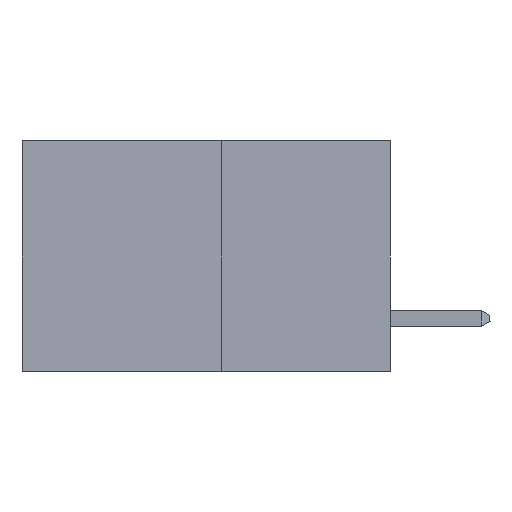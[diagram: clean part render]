
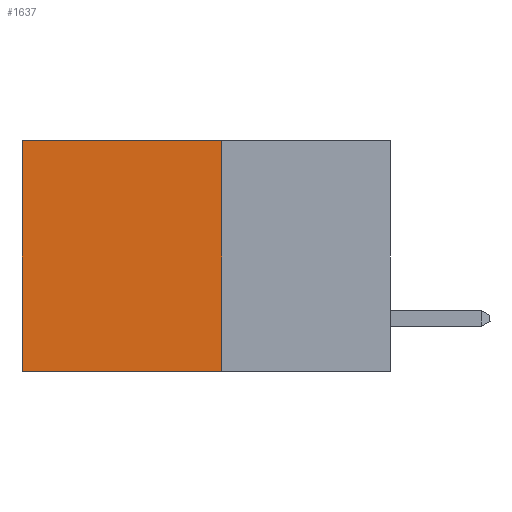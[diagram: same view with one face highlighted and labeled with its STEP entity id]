
A CAD part, left-side view. The second image highlights one B-rep face of the part: STEP entity #1637.
In plain terms, the highlighted planar face has unit normal (-1, 0, 0).
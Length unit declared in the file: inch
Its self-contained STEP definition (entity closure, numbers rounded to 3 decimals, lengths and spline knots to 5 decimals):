
#63 = EDGE_CURVE ( 'NONE', #3981, #15127, #5803, .T. ) ;
#303 = VERTEX_POINT ( 'NONE', #14389 ) ;
#711 = VECTOR ( 'NONE', #12782, 39.37008 ) ;
#761 = EDGE_LOOP ( 'NONE', ( #2103, #2134, #8928, #1982 ) ) ;
#1408 = PLANE ( 'NONE',  #7866 ) ;
#1637 = ADVANCED_FACE ( 'NONE', ( #5552 ), #1408, .F. ) ;
#1967 = VECTOR ( 'NONE', #15109, 39.37008 ) ;
#1982 = ORIENTED_EDGE ( 'NONE', *, *, #3085, .T. ) ;
#2053 = CARTESIAN_POINT ( 'NONE',  ( 0.277, 0.27, -0.37 ) ) ;
#2103 = ORIENTED_EDGE ( 'NONE', *, *, #63, .T. ) ;
#2134 = ORIENTED_EDGE ( 'NONE', *, *, #8322, .F. ) ;
#2957 = EDGE_CURVE ( 'NONE', #303, #5898, #11823, .T. ) ;
#3085 = EDGE_CURVE ( 'NONE', #303, #3981, #9901, .T. ) ;
#3717 = LINE ( 'NONE', #12818, #711 ) ;
#3981 = VERTEX_POINT ( 'NONE', #5483 ) ;
#5483 = CARTESIAN_POINT ( 'NONE',  ( 0.277, 0.59, 0. ) ) ;
#5552 = FACE_OUTER_BOUND ( 'NONE', #761, .T. ) ;
#5803 = LINE ( 'NONE', #7861, #15001 ) ;
#5898 = VERTEX_POINT ( 'NONE', #12848 ) ;
#5932 = CARTESIAN_POINT ( 'NONE',  ( 0.277, 0.27, -0.37 ) ) ;
#6012 = DIRECTION ( 'NONE',  ( 0., 1., 0. ) ) ;
#6507 = VECTOR ( 'NONE', #6012, 39.37008 ) ;
#7861 = CARTESIAN_POINT ( 'NONE',  ( 0.277, 0.59, -0.37 ) ) ;
#7866 = AXIS2_PLACEMENT_3D ( 'NONE', #2053, #11630, #11381 ) ;
#8322 = EDGE_CURVE ( 'NONE', #5898, #15127, #3717, .T. ) ;
#8928 = ORIENTED_EDGE ( 'NONE', *, *, #2957, .F. ) ;
#9416 = CARTESIAN_POINT ( 'NONE',  ( 0.277, 0.27, 0. ) ) ;
#9600 = CARTESIAN_POINT ( 'NONE',  ( 0.277, 0.59, -0.37 ) ) ;
#9901 = LINE ( 'NONE', #9416, #6507 ) ;
#11381 = DIRECTION ( 'NONE',  ( 0., 0., -1. ) ) ;
#11414 = DIRECTION ( 'NONE',  ( 0., 0., -1. ) ) ;
#11630 = DIRECTION ( 'NONE',  ( 1., 0., 0. ) ) ;
#11823 = LINE ( 'NONE', #5932, #1967 ) ;
#12782 = DIRECTION ( 'NONE',  ( 0., 1., 0. ) ) ;
#12818 = CARTESIAN_POINT ( 'NONE',  ( 0.277, 0.27, -0.37 ) ) ;
#12848 = CARTESIAN_POINT ( 'NONE',  ( 0.277, 0.27, -0.37 ) ) ;
#14389 = CARTESIAN_POINT ( 'NONE',  ( 0.277, 0.27, 0. ) ) ;
#15001 = VECTOR ( 'NONE', #11414, 39.37008 ) ;
#15109 = DIRECTION ( 'NONE',  ( 0., 0., -1. ) ) ;
#15127 = VERTEX_POINT ( 'NONE', #9600 ) ;
